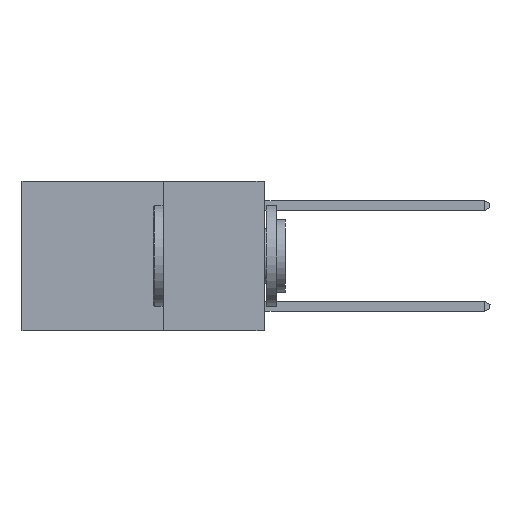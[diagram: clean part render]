
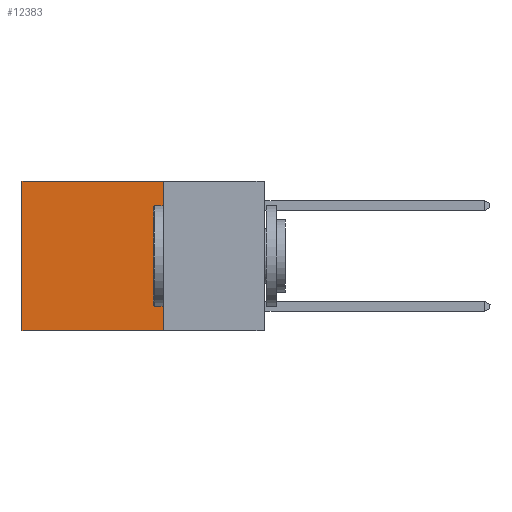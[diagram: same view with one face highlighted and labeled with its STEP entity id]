
A CAD part, left-side view. The second image highlights one B-rep face of the part: STEP entity #12383.
In plain terms, the highlighted planar face has unit normal (-1, 0, 0).
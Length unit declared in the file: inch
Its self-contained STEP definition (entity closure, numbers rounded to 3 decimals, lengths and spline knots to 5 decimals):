
#607 = CARTESIAN_POINT ( 'NONE',  ( 0.2625, 0.25, 0. ) ) ;
#1277 = PLANE ( 'NONE',  #17637 ) ;
#2889 = CARTESIAN_POINT ( 'NONE',  ( 0.2625, 0.6, 0. ) ) ;
#3231 = ORIENTED_EDGE ( 'NONE', *, *, #17358, .T. ) ;
#3408 = VERTEX_POINT ( 'NONE', #4462 ) ;
#4462 = CARTESIAN_POINT ( 'NONE',  ( 0.2625, 0.6, -0.37 ) ) ;
#5142 = CARTESIAN_POINT ( 'NONE',  ( 0.2625, 0.6, 0. ) ) ;
#5428 = FACE_OUTER_BOUND ( 'NONE', #6300, .T. ) ;
#6109 = ORIENTED_EDGE ( 'NONE', *, *, #6476, .T. ) ;
#6300 = EDGE_LOOP ( 'NONE', ( #6109, #17726, #14090, #3231 ) ) ;
#6476 = EDGE_CURVE ( 'NONE', #7302, #3408, #16345, .T. ) ;
#6517 = DIRECTION ( 'NONE',  ( 0., 0., -1. ) ) ;
#6793 = EDGE_CURVE ( 'NONE', #10765, #3408, #14307, .T. ) ;
#6822 = CARTESIAN_POINT ( 'NONE',  ( 0.2625, 0.25, 0. ) ) ;
#7156 = DIRECTION ( 'NONE',  ( 0., 1., 0. ) ) ;
#7197 = VECTOR ( 'NONE', #13289, 39.37008 ) ;
#7302 = VERTEX_POINT ( 'NONE', #2889 ) ;
#7352 = VECTOR ( 'NONE', #7156, 39.37008 ) ;
#8928 = VECTOR ( 'NONE', #13480, 39.37008 ) ;
#8985 = LINE ( 'NONE', #607, #7197 ) ;
#10473 = CARTESIAN_POINT ( 'NONE',  ( 0.2625, 0.25, 0. ) ) ;
#10513 = VERTEX_POINT ( 'NONE', #6822 ) ;
#10730 = DIRECTION ( 'NONE',  ( 1., 0., 0. ) ) ;
#10765 = VERTEX_POINT ( 'NONE', #17253 ) ;
#12383 = ADVANCED_FACE ( 'NONE', ( #5428 ), #1277, .F. ) ;
#13118 = LINE ( 'NONE', #10473, #8928 ) ;
#13289 = DIRECTION ( 'NONE',  ( 0., 1., 0. ) ) ;
#13480 = DIRECTION ( 'NONE',  ( 0., 0., -1. ) ) ;
#13571 = CARTESIAN_POINT ( 'NONE',  ( 0.2625, 0.25, 0. ) ) ;
#14090 = ORIENTED_EDGE ( 'NONE', *, *, #16881, .F. ) ;
#14307 = LINE ( 'NONE', #15674, #7352 ) ;
#14352 = VECTOR ( 'NONE', #6517, 39.37008 ) ;
#15674 = CARTESIAN_POINT ( 'NONE',  ( 0.2625, 0.25, -0.37 ) ) ;
#16345 = LINE ( 'NONE', #5142, #14352 ) ;
#16352 = DIRECTION ( 'NONE',  ( 0., 0., -1. ) ) ;
#16881 = EDGE_CURVE ( 'NONE', #10513, #10765, #13118, .T. ) ;
#17253 = CARTESIAN_POINT ( 'NONE',  ( 0.2625, 0.25, -0.37 ) ) ;
#17358 = EDGE_CURVE ( 'NONE', #10513, #7302, #8985, .T. ) ;
#17637 = AXIS2_PLACEMENT_3D ( 'NONE', #13571, #10730, #16352 ) ;
#17726 = ORIENTED_EDGE ( 'NONE', *, *, #6793, .F. ) ;
